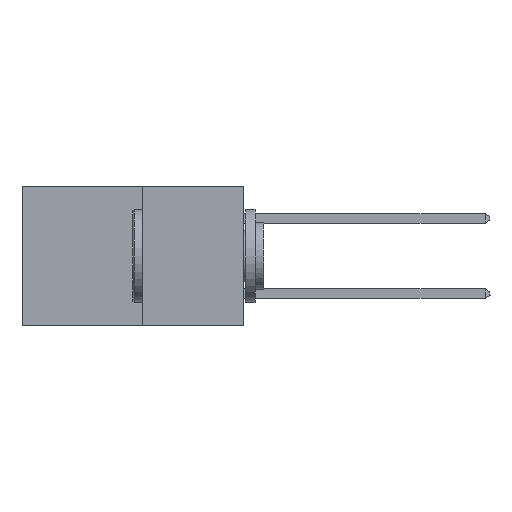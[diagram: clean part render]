
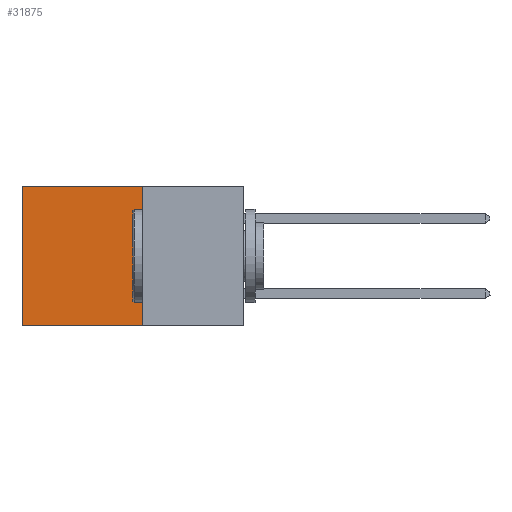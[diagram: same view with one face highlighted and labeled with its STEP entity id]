
A CAD part, left-side view. The second image highlights one B-rep face of the part: STEP entity #31875.
In plain terms, the highlighted planar face has unit normal (-1, 0, 0).
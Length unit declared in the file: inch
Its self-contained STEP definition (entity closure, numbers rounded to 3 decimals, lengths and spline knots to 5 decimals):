
#454 = LINE ( 'NONE', #9047, #19617 ) ;
#817 = VERTEX_POINT ( 'NONE', #31585 ) ;
#2457 = LINE ( 'NONE', #3571, #9140 ) ;
#3006 = DIRECTION ( 'NONE',  ( 0., 0., -1. ) ) ;
#3571 = CARTESIAN_POINT ( 'NONE',  ( 0.277, 0.27, 0. ) ) ;
#4544 = CARTESIAN_POINT ( 'NONE',  ( 0.277, 0.59, -0.37 ) ) ;
#6061 = EDGE_CURVE ( 'NONE', #23601, #14443, #7612, .T. ) ;
#6075 = CARTESIAN_POINT ( 'NONE',  ( 0.277, 0.27, -0.37 ) ) ;
#6725 = DIRECTION ( 'NONE',  ( 0., 1., 0. ) ) ;
#7256 = PLANE ( 'NONE',  #14830 ) ;
#7612 = LINE ( 'NONE', #6075, #20079 ) ;
#8235 = VECTOR ( 'NONE', #3006, 39.37008 ) ;
#9047 = CARTESIAN_POINT ( 'NONE',  ( 0.277, 0.59, -0.37 ) ) ;
#9140 = VECTOR ( 'NONE', #20998, 39.37008 ) ;
#9768 = CARTESIAN_POINT ( 'NONE',  ( 0.277, 0.27, -0.37 ) ) ;
#10603 = ORIENTED_EDGE ( 'NONE', *, *, #6061, .F. ) ;
#11515 = EDGE_CURVE ( 'NONE', #15581, #817, #2457, .T. ) ;
#12226 = DIRECTION ( 'NONE',  ( 0., 0., -1. ) ) ;
#13391 = EDGE_CURVE ( 'NONE', #15581, #23601, #20692, .T. ) ;
#14443 = VERTEX_POINT ( 'NONE', #4544 ) ;
#14830 = AXIS2_PLACEMENT_3D ( 'NONE', #9768, #27146, #12226 ) ;
#15581 = VERTEX_POINT ( 'NONE', #25792 ) ;
#16280 = EDGE_CURVE ( 'NONE', #817, #14443, #454, .T. ) ;
#19617 = VECTOR ( 'NONE', #23932, 39.37008 ) ;
#19770 = FACE_OUTER_BOUND ( 'NONE', #31082, .T. ) ;
#20079 = VECTOR ( 'NONE', #6725, 39.37008 ) ;
#20692 = LINE ( 'NONE', #27849, #8235 ) ;
#20998 = DIRECTION ( 'NONE',  ( 0., 1., 0. ) ) ;
#21040 = ORIENTED_EDGE ( 'NONE', *, *, #13391, .F. ) ;
#22054 = CARTESIAN_POINT ( 'NONE',  ( 0.277, 0.27, -0.37 ) ) ;
#23601 = VERTEX_POINT ( 'NONE', #22054 ) ;
#23932 = DIRECTION ( 'NONE',  ( 0., 0., -1. ) ) ;
#24793 = ORIENTED_EDGE ( 'NONE', *, *, #16280, .T. ) ;
#25792 = CARTESIAN_POINT ( 'NONE',  ( 0.277, 0.27, 0. ) ) ;
#26949 = ORIENTED_EDGE ( 'NONE', *, *, #11515, .T. ) ;
#27146 = DIRECTION ( 'NONE',  ( 1., 0., 0. ) ) ;
#27849 = CARTESIAN_POINT ( 'NONE',  ( 0.277, 0.27, -0.37 ) ) ;
#31082 = EDGE_LOOP ( 'NONE', ( #24793, #10603, #21040, #26949 ) ) ;
#31585 = CARTESIAN_POINT ( 'NONE',  ( 0.277, 0.59, 0. ) ) ;
#31875 = ADVANCED_FACE ( 'NONE', ( #19770 ), #7256, .F. ) ;
